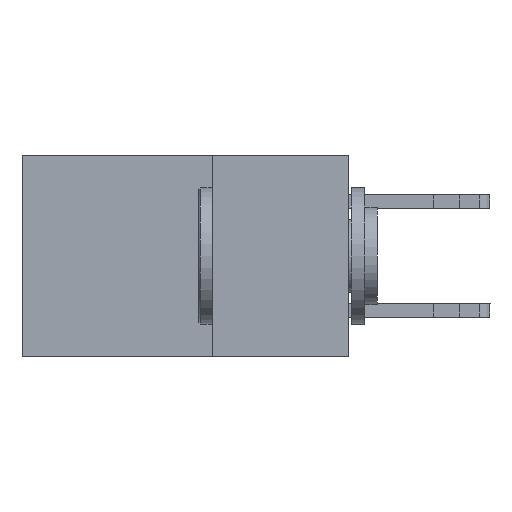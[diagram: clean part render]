
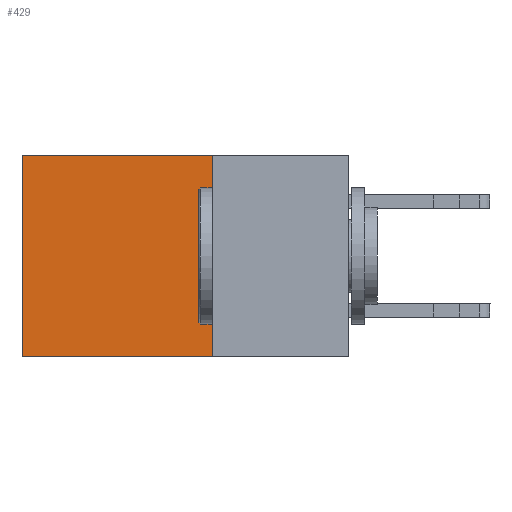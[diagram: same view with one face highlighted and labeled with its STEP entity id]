
A CAD part, left-side view. The second image highlights one B-rep face of the part: STEP entity #429.
In plain terms, the highlighted planar face has unit normal (-1, 0, 0).
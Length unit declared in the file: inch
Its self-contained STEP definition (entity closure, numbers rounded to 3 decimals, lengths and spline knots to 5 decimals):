
#210 = EDGE_CURVE ( 'NONE', #10513, #19834, #20295, .T. ) ;
#429 = ADVANCED_FACE ( 'NONE', ( #14131 ), #23838, .F. ) ;
#1038 = CARTESIAN_POINT ( 'NONE',  ( 0.298, 0.6, 0. ) ) ;
#1682 = EDGE_CURVE ( 'NONE', #8710, #10513, #7937, .T. ) ;
#2044 = DIRECTION ( 'NONE',  ( 0., 1., 0. ) ) ;
#2737 = VECTOR ( 'NONE', #14933, 39.37008 ) ;
#4271 = CARTESIAN_POINT ( 'NONE',  ( 0.298, 0.25, 0. ) ) ;
#5588 = CARTESIAN_POINT ( 'NONE',  ( 0.298, 0.25, -0.37 ) ) ;
#5875 = CARTESIAN_POINT ( 'NONE',  ( 0.298, 0.25, 0. ) ) ;
#6240 = DIRECTION ( 'NONE',  ( 1., 0., 0. ) ) ;
#6881 = CARTESIAN_POINT ( 'NONE',  ( 0.298, 0.25, 0. ) ) ;
#7079 = VECTOR ( 'NONE', #2044, 39.37008 ) ;
#7937 = LINE ( 'NONE', #23825, #11286 ) ;
#8710 = VERTEX_POINT ( 'NONE', #5875 ) ;
#8790 = DIRECTION ( 'NONE',  ( 0., 0., -1. ) ) ;
#8975 = EDGE_LOOP ( 'NONE', ( #14760, #10408, #24267, #16687 ) ) ;
#9922 = VECTOR ( 'NONE', #10991, 39.37008 ) ;
#9931 = CARTESIAN_POINT ( 'NONE',  ( 0.298, 0.25, -0.37 ) ) ;
#10408 = ORIENTED_EDGE ( 'NONE', *, *, #210, .F. ) ;
#10513 = VERTEX_POINT ( 'NONE', #5588 ) ;
#10991 = DIRECTION ( 'NONE',  ( 0., 1., 0. ) ) ;
#11286 = VECTOR ( 'NONE', #15849, 39.37008 ) ;
#13681 = CARTESIAN_POINT ( 'NONE',  ( 0.298, 0.6, 0. ) ) ;
#14131 = FACE_OUTER_BOUND ( 'NONE', #8975, .T. ) ;
#14707 = VERTEX_POINT ( 'NONE', #13681 ) ;
#14760 = ORIENTED_EDGE ( 'NONE', *, *, #22274, .T. ) ;
#14933 = DIRECTION ( 'NONE',  ( 0., 0., -1. ) ) ;
#15849 = DIRECTION ( 'NONE',  ( 0., 0., -1. ) ) ;
#16615 = CARTESIAN_POINT ( 'NONE',  ( 0.298, 0.6, -0.37 ) ) ;
#16687 = ORIENTED_EDGE ( 'NONE', *, *, #20135, .T. ) ;
#18820 = AXIS2_PLACEMENT_3D ( 'NONE', #4271, #6240, #8790 ) ;
#19834 = VERTEX_POINT ( 'NONE', #16615 ) ;
#20135 = EDGE_CURVE ( 'NONE', #8710, #14707, #22228, .T. ) ;
#20295 = LINE ( 'NONE', #9931, #7079 ) ;
#21177 = LINE ( 'NONE', #1038, #2737 ) ;
#22228 = LINE ( 'NONE', #6881, #9922 ) ;
#22274 = EDGE_CURVE ( 'NONE', #14707, #19834, #21177, .T. ) ;
#23825 = CARTESIAN_POINT ( 'NONE',  ( 0.298, 0.25, 0. ) ) ;
#23838 = PLANE ( 'NONE',  #18820 ) ;
#24267 = ORIENTED_EDGE ( 'NONE', *, *, #1682, .F. ) ;
